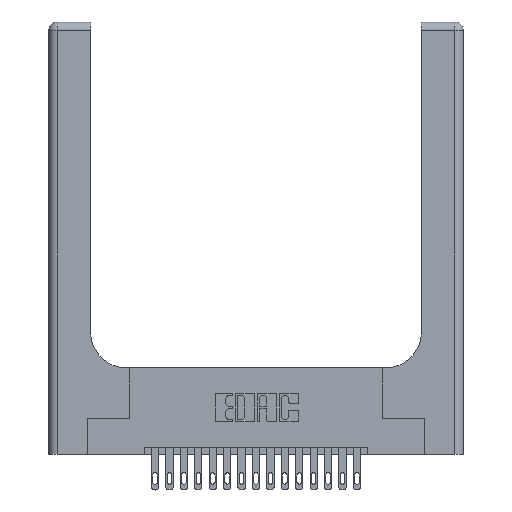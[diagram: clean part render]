
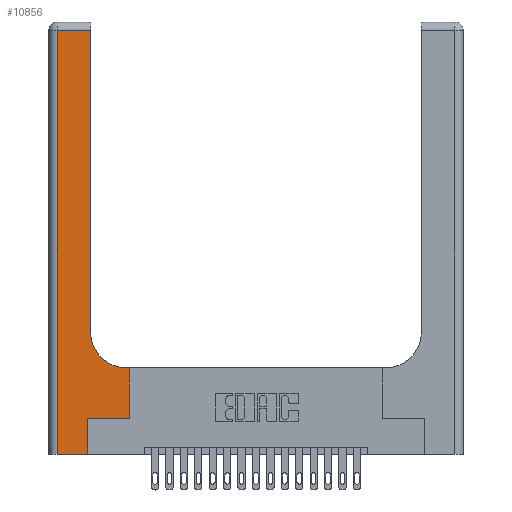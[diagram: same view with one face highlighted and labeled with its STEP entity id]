
A CAD part, top view. The second image highlights one B-rep face of the part: STEP entity #10856.
In plain terms, the highlighted planar face has unit normal (0, 0, 1).
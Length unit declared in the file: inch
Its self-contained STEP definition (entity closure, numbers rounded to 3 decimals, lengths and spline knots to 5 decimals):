
#435 = VERTEX_POINT ( 'NONE', #14784 ) ;
#501 = DIRECTION ( 'NONE',  ( 0., 0., -1. ) ) ;
#1758 = CARTESIAN_POINT ( 'NONE',  ( 0.269, 0., 0.37 ) ) ;
#1961 = VERTEX_POINT ( 'NONE', #5667 ) ;
#2451 = CARTESIAN_POINT ( 'NONE',  ( 0.269, 0., 0.37 ) ) ;
#2688 = DIRECTION ( 'NONE',  ( 1., 0., 0. ) ) ;
#2731 = DIRECTION ( 'NONE',  ( 0., 1., 0. ) ) ;
#2986 = ORIENTED_EDGE ( 'NONE', *, *, #15307, .T. ) ;
#3186 = CARTESIAN_POINT ( 'NONE',  ( 0.5585, 0.25, 0.37 ) ) ;
#3854 = VECTOR ( 'NONE', #19623, 39.37008 ) ;
#4436 = CIRCLE ( 'NONE', #6977, 0.25 ) ;
#4539 = EDGE_CURVE ( 'NONE', #6956, #9614, #15930, .T. ) ;
#5242 = LINE ( 'NONE', #14280, #7715 ) ;
#5667 = CARTESIAN_POINT ( 'NONE',  ( 0.2915, 0.85, 0.37 ) ) ;
#5774 = EDGE_LOOP ( 'NONE', ( #7969, #7412, #2986, #7892, #15396, #15073, #6230, #11667, #13007 ) ) ;
#6230 = ORIENTED_EDGE ( 'NONE', *, *, #13813, .T. ) ;
#6947 = DIRECTION ( 'NONE',  ( -1., 0., 0. ) ) ;
#6956 = VERTEX_POINT ( 'NONE', #1758 ) ;
#6977 = AXIS2_PLACEMENT_3D ( 'NONE', #11640, #13235, #18116 ) ;
#7399 = VECTOR ( 'NONE', #13405, 39.37008 ) ;
#7412 = ORIENTED_EDGE ( 'NONE', *, *, #18331, .T. ) ;
#7539 = CARTESIAN_POINT ( 'NONE',  ( 0.2915, 3., 0.37 ) ) ;
#7715 = VECTOR ( 'NONE', #15899, 39.37008 ) ;
#7892 = ORIENTED_EDGE ( 'NONE', *, *, #17769, .T. ) ;
#7969 = ORIENTED_EDGE ( 'NONE', *, *, #17930, .T. ) ;
#8564 = CARTESIAN_POINT ( 'NONE',  ( 0., 2.94, 0.37 ) ) ;
#8866 = DIRECTION ( 'NONE',  ( -1., 0., 0. ) ) ;
#9614 = VERTEX_POINT ( 'NONE', #10915 ) ;
#9790 = CARTESIAN_POINT ( 'NONE',  ( 0.06, 2.94, 0.37 ) ) ;
#9875 = LINE ( 'NONE', #15008, #7399 ) ;
#9945 = EDGE_CURVE ( 'NONE', #9614, #18907, #11800, .T. ) ;
#10522 = CARTESIAN_POINT ( 'NONE',  ( 0.5415, 0.6, 0.37 ) ) ;
#10856 = ADVANCED_FACE ( 'NONE', ( #20453 ), #16449, .F. ) ;
#10915 = CARTESIAN_POINT ( 'NONE',  ( 0.269, 0.25, 0.37 ) ) ;
#10917 = EDGE_CURVE ( 'NONE', #15816, #14676, #13254, .T. ) ;
#11640 = CARTESIAN_POINT ( 'NONE',  ( 0.5415, 0.85, 0.37 ) ) ;
#11667 = ORIENTED_EDGE ( 'NONE', *, *, #10917, .T. ) ;
#11800 = LINE ( 'NONE', #20211, #16282 ) ;
#12286 = LINE ( 'NONE', #8564, #3854 ) ;
#12458 = CARTESIAN_POINT ( 'NONE',  ( 0.2915, 2.94, 0.37 ) ) ;
#12665 = VERTEX_POINT ( 'NONE', #9790 ) ;
#13007 = ORIENTED_EDGE ( 'NONE', *, *, #14573, .T. ) ;
#13235 = DIRECTION ( 'NONE',  ( 0., 0., -1. ) ) ;
#13254 = LINE ( 'NONE', #14910, #17997 ) ;
#13405 = DIRECTION ( 'NONE',  ( 0., -1., 0. ) ) ;
#13813 = EDGE_CURVE ( 'NONE', #18907, #15816, #5242, .T. ) ;
#14280 = CARTESIAN_POINT ( 'NONE',  ( 0.5585, 0.25, 0.37 ) ) ;
#14535 = LINE ( 'NONE', #7539, #19293 ) ;
#14573 = EDGE_CURVE ( 'NONE', #14676, #1961, #4436, .T. ) ;
#14676 = VERTEX_POINT ( 'NONE', #10522 ) ;
#14784 = CARTESIAN_POINT ( 'NONE',  ( 0.06, 0., 0.37 ) ) ;
#14848 = VERTEX_POINT ( 'NONE', #12458 ) ;
#14880 = AXIS2_PLACEMENT_3D ( 'NONE', #16177, #501, #6947 ) ;
#14910 = CARTESIAN_POINT ( 'NONE',  ( 0.2915, 0.6, 0.37 ) ) ;
#15008 = CARTESIAN_POINT ( 'NONE',  ( 0.06, 3., 0.37 ) ) ;
#15073 = ORIENTED_EDGE ( 'NONE', *, *, #9945, .T. ) ;
#15307 = EDGE_CURVE ( 'NONE', #12665, #435, #9875, .T. ) ;
#15396 = ORIENTED_EDGE ( 'NONE', *, *, #4539, .T. ) ;
#15421 = VECTOR ( 'NONE', #18355, 39.37008 ) ;
#15816 = VERTEX_POINT ( 'NONE', #19475 ) ;
#15899 = DIRECTION ( 'NONE',  ( 0., 1., 0. ) ) ;
#15930 = LINE ( 'NONE', #2451, #15421 ) ;
#16177 = CARTESIAN_POINT ( 'NONE',  ( 0., 3., 0.37 ) ) ;
#16282 = VECTOR ( 'NONE', #2688, 39.37008 ) ;
#16449 = PLANE ( 'NONE',  #14880 ) ;
#17281 = LINE ( 'NONE', #17762, #18285 ) ;
#17762 = CARTESIAN_POINT ( 'NONE',  ( 0., 0., 0.37 ) ) ;
#17769 = EDGE_CURVE ( 'NONE', #435, #6956, #17281, .T. ) ;
#17930 = EDGE_CURVE ( 'NONE', #1961, #14848, #14535, .T. ) ;
#17997 = VECTOR ( 'NONE', #8866, 39.37008 ) ;
#18116 = DIRECTION ( 'NONE',  ( 1., 0., 0. ) ) ;
#18285 = VECTOR ( 'NONE', #19514, 39.37008 ) ;
#18331 = EDGE_CURVE ( 'NONE', #14848, #12665, #12286, .T. ) ;
#18355 = DIRECTION ( 'NONE',  ( 0., 1., 0. ) ) ;
#18907 = VERTEX_POINT ( 'NONE', #3186 ) ;
#19293 = VECTOR ( 'NONE', #2731, 39.37008 ) ;
#19475 = CARTESIAN_POINT ( 'NONE',  ( 0.5585, 0.6, 0.37 ) ) ;
#19514 = DIRECTION ( 'NONE',  ( 1., 0., 0. ) ) ;
#19623 = DIRECTION ( 'NONE',  ( -1., 0., 0. ) ) ;
#20211 = CARTESIAN_POINT ( 'NONE',  ( 0.269, 0.25, 0.37 ) ) ;
#20453 = FACE_OUTER_BOUND ( 'NONE', #5774, .T. ) ;
